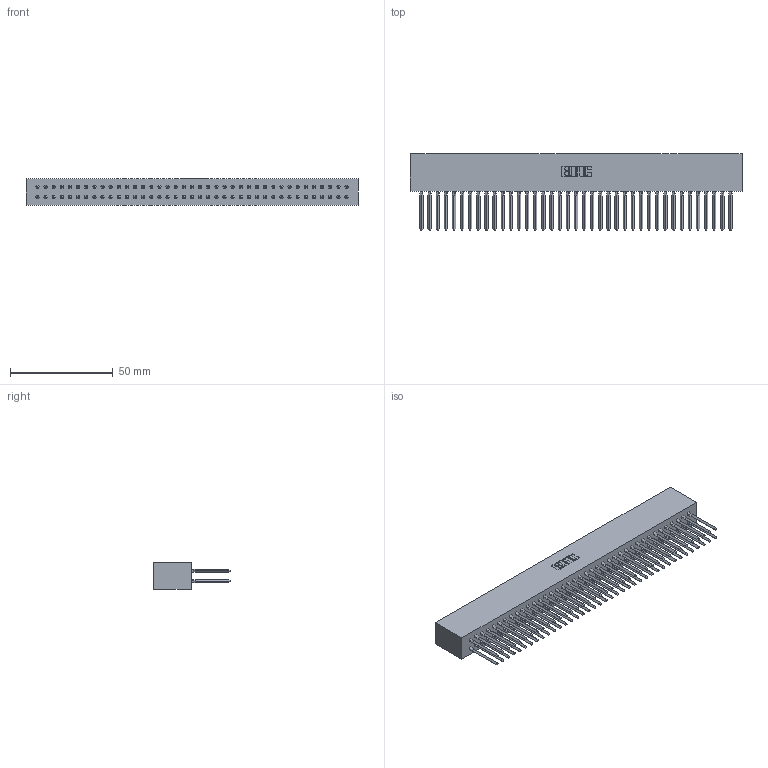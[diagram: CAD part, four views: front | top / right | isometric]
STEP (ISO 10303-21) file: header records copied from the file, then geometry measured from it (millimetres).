
FILE_DESCRIPTION (( 'STEP AP203' ), '1' );
FILE_NAME ('317-078-540-801.STEP', '2020-02-28T08:37:52', ( '' ), ( '' ), 'SwSTEP 2.0', 'SolidWorks 2016', '' );
FILE_SCHEMA (( 'CONFIG_CONTROL_DESIGN' ));
Length unit declared in the file: inch
Products named in the file (3): 317-290-001_540; 317-078-540-801; 317 Part_Lugless
Assembly tree (79 placements, depth 2):
  317-078-540-801
    317 Part_Lugless
    317-290-001_540  x78
Bounding box: 161.75 x 37.34 x 12.7 mm (x, y, z)
Volume: 28838.3 mm3; surface area: 43138.9 mm2
Topology: 79 solids, 79 shells, 7032 faces, 19505 edges, 12560 vertices
Faces by surface type: plane 5744, cylinder 976, bspline 312
Entity records: 56384 total; most frequent: CARTESIAN_POINT 10251, ORIENTED_EDGE 9750, DIRECTION 8125, EDGE_CURVE 4875, LINE 4627, VECTOR 4627, VERTEX_POINT 3243, AXIS2_PLACEMENT_3D 1749
